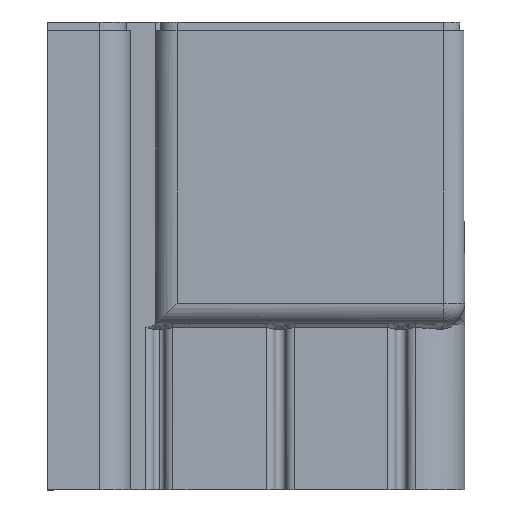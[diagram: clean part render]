
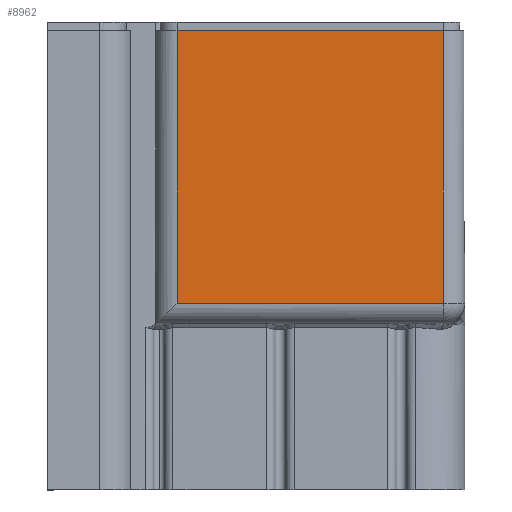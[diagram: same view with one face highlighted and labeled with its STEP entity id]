
A CAD part, left-side view. The second image highlights one B-rep face of the part: STEP entity #8962.
In plain terms, the highlighted planar face has unit normal (-1, 0, 0).
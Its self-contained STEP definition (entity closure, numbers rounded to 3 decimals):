
#167 = EDGE_LOOP ( 'NONE', ( #6127, #6121, #6055, #6308 ) ) ;
#406 = CARTESIAN_POINT ( 'NONE',  ( -167.726, -127.293, -14.394 ) ) ;
#528 = VECTOR ( 'NONE', #2536, 1000. ) ;
#1098 = VERTEX_POINT ( 'NONE', #5105 ) ;
#1310 = VERTEX_POINT ( 'NONE', #4016 ) ;
#1403 = VECTOR ( 'NONE', #1974, 1000. ) ;
#1697 = CARTESIAN_POINT ( 'NONE',  ( -167.726, -94.588, -14.394 ) ) ;
#1974 = DIRECTION ( 'NONE',  ( 0., -1., 0. ) ) ;
#2166 = FACE_OUTER_BOUND ( 'NONE', #167, .T. ) ;
#2536 = DIRECTION ( 'NONE',  ( 0., 0., 1. ) ) ;
#4016 = CARTESIAN_POINT ( 'NONE',  ( -167.726, -33.201, 48.505 ) ) ;
#4386 = CARTESIAN_POINT ( 'NONE',  ( -167.726, -33.201, -19.394 ) ) ;
#4924 = AXIS2_PLACEMENT_3D ( 'NONE', #5136, #8494, #6598 ) ;
#5095 = DIRECTION ( 'NONE',  ( 0., -1., 0. ) ) ;
#5105 = CARTESIAN_POINT ( 'NONE',  ( -167.726, -94.588, 48.505 ) ) ;
#5136 = CARTESIAN_POINT ( 'NONE',  ( -167.726, -127.293, -19.394 ) ) ;
#5292 = LINE ( 'NONE', #406, #7784 ) ;
#5422 = VERTEX_POINT ( 'NONE', #6706 ) ;
#5510 = LINE ( 'NONE', #8430, #1403 ) ;
#5877 = PLANE ( 'NONE',  #4924 ) ;
#5900 = DIRECTION ( 'NONE',  ( 0., 0., -1. ) ) ;
#6055 = ORIENTED_EDGE ( 'NONE', *, *, #6744, .T. ) ;
#6121 = ORIENTED_EDGE ( 'NONE', *, *, #6409, .T. ) ;
#6127 = ORIENTED_EDGE ( 'NONE', *, *, #6729, .F. ) ;
#6308 = ORIENTED_EDGE ( 'NONE', *, *, #6543, .T. ) ;
#6409 = EDGE_CURVE ( 'NONE', #1310, #5422, #9111, .T. ) ;
#6543 = EDGE_CURVE ( 'NONE', #8269, #1098, #8168, .T. ) ;
#6598 = DIRECTION ( 'NONE',  ( 0., 0., -1. ) ) ;
#6706 = CARTESIAN_POINT ( 'NONE',  ( -167.726, -33.201, -14.394 ) ) ;
#6729 = EDGE_CURVE ( 'NONE', #1310, #1098, #5510, .T. ) ;
#6744 = EDGE_CURVE ( 'NONE', #5422, #8269, #5292, .T. ) ;
#7694 = CARTESIAN_POINT ( 'NONE',  ( -167.726, -94.588, -19.394 ) ) ;
#7784 = VECTOR ( 'NONE', #5095, 1000. ) ;
#8168 = LINE ( 'NONE', #7694, #528 ) ;
#8269 = VERTEX_POINT ( 'NONE', #1697 ) ;
#8430 = CARTESIAN_POINT ( 'NONE',  ( -167.726, -127.293, 48.505 ) ) ;
#8494 = DIRECTION ( 'NONE',  ( 1., 0., 0. ) ) ;
#8962 = ADVANCED_FACE ( 'NONE', ( #2166 ), #5877, .F. ) ;
#9111 = LINE ( 'NONE', #4386, #9294 ) ;
#9294 = VECTOR ( 'NONE', #5900, 1000. ) ;
